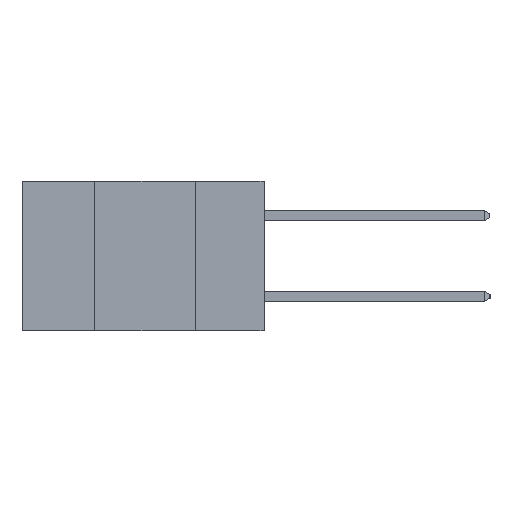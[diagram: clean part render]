
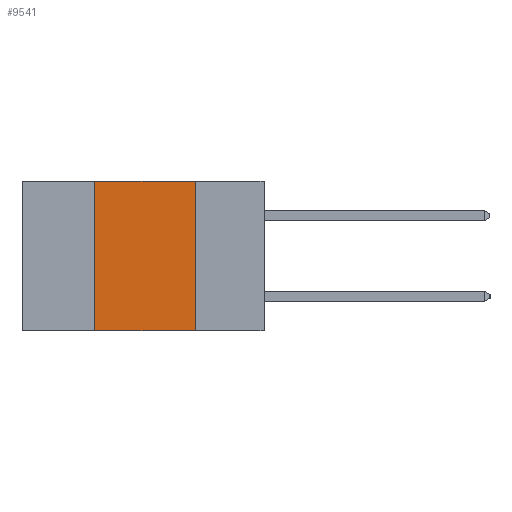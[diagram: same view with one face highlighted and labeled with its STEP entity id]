
A CAD part, left-side view. The second image highlights one B-rep face of the part: STEP entity #9541.
In plain terms, the highlighted planar face has unit normal (-1, 0, 0).
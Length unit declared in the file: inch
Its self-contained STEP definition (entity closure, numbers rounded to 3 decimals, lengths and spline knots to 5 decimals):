
#13 = CARTESIAN_POINT ( 'NONE',  ( 0., 0.42, -0.37 ) ) ;
#62 = ORIENTED_EDGE ( 'NONE', *, *, #13538, .F. ) ;
#1009 = VERTEX_POINT ( 'NONE', #15760 ) ;
#1727 = DIRECTION ( 'NONE',  ( 0., -1., 0. ) ) ;
#1861 = CARTESIAN_POINT ( 'NONE',  ( 0., 0.6, -0.37 ) ) ;
#2301 = VECTOR ( 'NONE', #12760, 39.37008 ) ;
#3360 = VERTEX_POINT ( 'NONE', #14915 ) ;
#4723 = CARTESIAN_POINT ( 'NONE',  ( 0., 0.17, 0. ) ) ;
#5231 = VECTOR ( 'NONE', #6709, 39.37008 ) ;
#6357 = LINE ( 'NONE', #6863, #9453 ) ;
#6582 = EDGE_CURVE ( 'NONE', #9103, #3360, #11692, .T. ) ;
#6709 = DIRECTION ( 'NONE',  ( 0., 0., -1. ) ) ;
#6863 = CARTESIAN_POINT ( 'NONE',  ( 0., 0.6, 0. ) ) ;
#6898 = EDGE_CURVE ( 'NONE', #9103, #1009, #11322, .T. ) ;
#7036 = EDGE_CURVE ( 'NONE', #1009, #12430, #6357, .T. ) ;
#7352 = DIRECTION ( 'NONE',  ( 0., -1., 0. ) ) ;
#7460 = CARTESIAN_POINT ( 'NONE',  ( 0., 0.17, -0.37 ) ) ;
#7627 = DIRECTION ( 'NONE',  ( 0., 0., -1. ) ) ;
#7705 = DIRECTION ( 'NONE',  ( 1., 0., 0. ) ) ;
#7753 = PLANE ( 'NONE',  #9111 ) ;
#7874 = CARTESIAN_POINT ( 'NONE',  ( 0., 0.6, 0. ) ) ;
#8737 = VECTOR ( 'NONE', #1727, 39.37008 ) ;
#9103 = VERTEX_POINT ( 'NONE', #13 ) ;
#9111 = AXIS2_PLACEMENT_3D ( 'NONE', #7874, #7705, #7627 ) ;
#9453 = VECTOR ( 'NONE', #7352, 39.37008 ) ;
#9541 = ADVANCED_FACE ( 'NONE', ( #13198 ), #7753, .F. ) ;
#11322 = LINE ( 'NONE', #12721, #2301 ) ;
#11692 = LINE ( 'NONE', #1861, #8737 ) ;
#11865 = ORIENTED_EDGE ( 'NONE', *, *, #6582, .T. ) ;
#12430 = VERTEX_POINT ( 'NONE', #4723 ) ;
#12721 = CARTESIAN_POINT ( 'NONE',  ( 0., 0.42, -0.37 ) ) ;
#12760 = DIRECTION ( 'NONE',  ( 0., 0., 1. ) ) ;
#13198 = FACE_OUTER_BOUND ( 'NONE', #13853, .T. ) ;
#13538 = EDGE_CURVE ( 'NONE', #12430, #3360, #14812, .T. ) ;
#13853 = EDGE_LOOP ( 'NONE', ( #62, #14323, #14704, #11865 ) ) ;
#14323 = ORIENTED_EDGE ( 'NONE', *, *, #7036, .F. ) ;
#14704 = ORIENTED_EDGE ( 'NONE', *, *, #6898, .F. ) ;
#14812 = LINE ( 'NONE', #7460, #5231 ) ;
#14915 = CARTESIAN_POINT ( 'NONE',  ( 0., 0.17, -0.37 ) ) ;
#15760 = CARTESIAN_POINT ( 'NONE',  ( 0., 0.42, 0. ) ) ;
